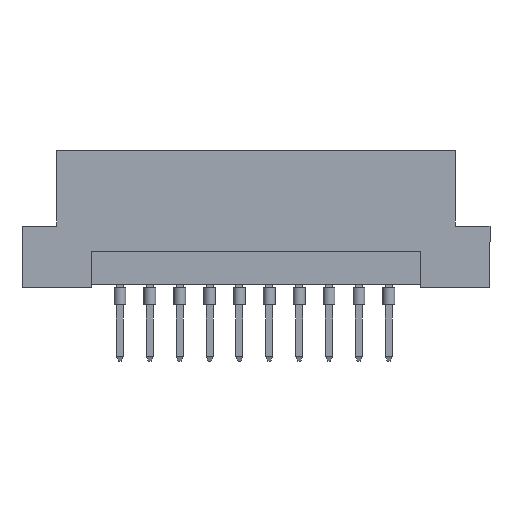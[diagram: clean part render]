
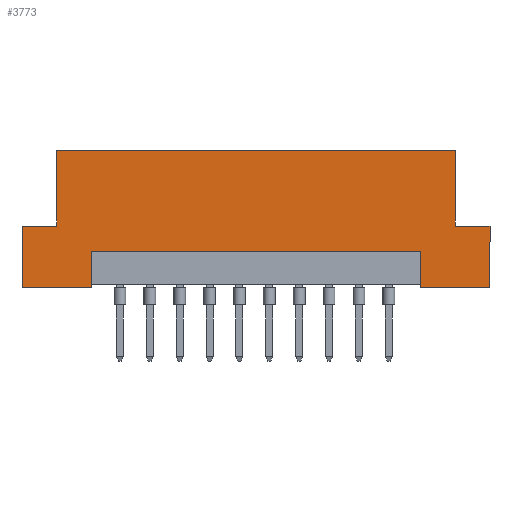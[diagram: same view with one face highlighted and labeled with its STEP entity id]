
A CAD part, front view. The second image highlights one B-rep face of the part: STEP entity #3773.
In plain terms, the highlighted planar face has unit normal (0, -1, 0).
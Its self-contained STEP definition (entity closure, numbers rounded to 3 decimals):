
#22 = VECTOR ( 'NONE', #2826, 1000. ) ;
#54 = LINE ( 'NONE', #463, #5178 ) ;
#62 = DIRECTION ( 'NONE',  ( 1., 0., 0. ) ) ;
#83 = ORIENTED_EDGE ( 'NONE', *, *, #1133, .F. ) ;
#179 = EDGE_CURVE ( 'NONE', #1130, #1898, #4204, .T. ) ;
#191 = ORIENTED_EDGE ( 'NONE', *, *, #2195, .T. ) ;
#226 = DIRECTION ( 'NONE',  ( 0., 0., 1. ) ) ;
#286 = CARTESIAN_POINT ( 'NONE',  ( 16.94, -4.3, 5.2 ) ) ;
#406 = VERTEX_POINT ( 'NONE', #3830 ) ;
#463 = CARTESIAN_POINT ( 'NONE',  ( 19.9, -4.3, 11.6 ) ) ;
#523 = EDGE_CURVE ( 'NONE', #3081, #2697, #657, .T. ) ;
#524 = DIRECTION ( 'NONE',  ( 1., 0., 0. ) ) ;
#594 = DIRECTION ( 'NONE',  ( 0., 0., -1. ) ) ;
#620 = ORIENTED_EDGE ( 'NONE', *, *, #4673, .F. ) ;
#657 = LINE ( 'NONE', #4878, #22 ) ;
#660 = CARTESIAN_POINT ( 'NONE',  ( 19.9, -4.3, 5.2 ) ) ;
#670 = DIRECTION ( 'NONE',  ( 0., 0., -1. ) ) ;
#687 = CARTESIAN_POINT ( 'NONE',  ( 14., -4.3, 3. ) ) ;
#706 = CARTESIAN_POINT ( 'NONE',  ( -14., -4.3, 3. ) ) ;
#811 = CARTESIAN_POINT ( 'NONE',  ( -19.9, -4.3, 11.6 ) ) ;
#885 = VECTOR ( 'NONE', #62, 1000. ) ;
#915 = CARTESIAN_POINT ( 'NONE',  ( -19.9, -4.3, 5.2 ) ) ;
#1026 = ORIENTED_EDGE ( 'NONE', *, *, #4464, .F. ) ;
#1111 = VECTOR ( 'NONE', #5130, 1000. ) ;
#1130 = VERTEX_POINT ( 'NONE', #2294 ) ;
#1133 = EDGE_CURVE ( 'NONE', #4198, #1898, #3945, .T. ) ;
#1314 = ORIENTED_EDGE ( 'NONE', *, *, #4512, .T. ) ;
#1452 = CARTESIAN_POINT ( 'NONE',  ( -14., -4.3, 3. ) ) ;
#1474 = CARTESIAN_POINT ( 'NONE',  ( -14., -4.3, 0.2 ) ) ;
#1511 = EDGE_LOOP ( 'NONE', ( #2979, #620, #3837, #4017, #2595, #1314, #2656, #1026, #4530, #191, #2821, #83 ) ) ;
#1546 = VECTOR ( 'NONE', #2391, 1000. ) ;
#1682 = LINE ( 'NONE', #4716, #4160 ) ;
#1689 = VERTEX_POINT ( 'NONE', #286 ) ;
#1718 = DIRECTION ( 'NONE',  ( 1., 0., 0. ) ) ;
#1791 = CARTESIAN_POINT ( 'NONE',  ( -14., -4.3, 0. ) ) ;
#1898 = VERTEX_POINT ( 'NONE', #1791 ) ;
#1913 = VECTOR ( 'NONE', #2459, 1000. ) ;
#1931 = EDGE_CURVE ( 'NONE', #1689, #4643, #1682, .T. ) ;
#2195 = EDGE_CURVE ( 'NONE', #5096, #1130, #4946, .T. ) ;
#2254 = DIRECTION ( 'NONE',  ( 1., 0., 0. ) ) ;
#2269 = LINE ( 'NONE', #4709, #4513 ) ;
#2283 = PLANE ( 'NONE',  #5342 ) ;
#2294 = CARTESIAN_POINT ( 'NONE',  ( -19.9, -4.3, 0. ) ) ;
#2307 = VECTOR ( 'NONE', #1718, 1000. ) ;
#2391 = DIRECTION ( 'NONE',  ( 0., 0., 1. ) ) ;
#2453 = EDGE_CURVE ( 'NONE', #4643, #2697, #2269, .T. ) ;
#2459 = DIRECTION ( 'NONE',  ( 0., 0., -1. ) ) ;
#2559 = CARTESIAN_POINT ( 'NONE',  ( -19.9, -4.3, 5.2 ) ) ;
#2595 = ORIENTED_EDGE ( 'NONE', *, *, #1931, .F. ) ;
#2656 = ORIENTED_EDGE ( 'NONE', *, *, #4054, .F. ) ;
#2697 = VERTEX_POINT ( 'NONE', #3244 ) ;
#2724 = EDGE_CURVE ( 'NONE', #5096, #3654, #3754, .T. ) ;
#2821 = ORIENTED_EDGE ( 'NONE', *, *, #179, .T. ) ;
#2826 = DIRECTION ( 'NONE',  ( 1., 0., 0. ) ) ;
#2829 = CARTESIAN_POINT ( 'NONE',  ( 16.94, -4.3, 11.6 ) ) ;
#2979 = ORIENTED_EDGE ( 'NONE', *, *, #3908, .T. ) ;
#3027 = CARTESIAN_POINT ( 'NONE',  ( 16.94, -4.3, 5.2 ) ) ;
#3081 = VERTEX_POINT ( 'NONE', #4157 ) ;
#3154 = DIRECTION ( 'NONE',  ( 0., 1., 0. ) ) ;
#3167 = DIRECTION ( 'NONE',  ( 1., 0., 0. ) ) ;
#3244 = CARTESIAN_POINT ( 'NONE',  ( 19.9, -4.3, 0. ) ) ;
#3277 = VECTOR ( 'NONE', #3167, 1000. ) ;
#3519 = LINE ( 'NONE', #1452, #3277 ) ;
#3533 = CARTESIAN_POINT ( 'NONE',  ( 19.9, -4.3, 11.6 ) ) ;
#3535 = LINE ( 'NONE', #3027, #1111 ) ;
#3654 = VERTEX_POINT ( 'NONE', #4823 ) ;
#3710 = VERTEX_POINT ( 'NONE', #687 ) ;
#3754 = LINE ( 'NONE', #2559, #2307 ) ;
#3773 = ADVANCED_FACE ( 'NONE', ( #4337 ), #2283, .F. ) ;
#3830 = CARTESIAN_POINT ( 'NONE',  ( -16.94, -4.3, 11.6 ) ) ;
#3834 = LINE ( 'NONE', #4646, #5097 ) ;
#3837 = ORIENTED_EDGE ( 'NONE', *, *, #523, .T. ) ;
#3908 = EDGE_CURVE ( 'NONE', #4198, #3710, #3519, .T. ) ;
#3945 = LINE ( 'NONE', #1474, #4516 ) ;
#4017 = ORIENTED_EDGE ( 'NONE', *, *, #2453, .F. ) ;
#4054 = EDGE_CURVE ( 'NONE', #406, #4619, #54, .T. ) ;
#4157 = CARTESIAN_POINT ( 'NONE',  ( 14., -4.3, 0. ) ) ;
#4160 = VECTOR ( 'NONE', #2254, 1000. ) ;
#4198 = VERTEX_POINT ( 'NONE', #706 ) ;
#4204 = LINE ( 'NONE', #5340, #885 ) ;
#4337 = FACE_OUTER_BOUND ( 'NONE', #1511, .T. ) ;
#4464 = EDGE_CURVE ( 'NONE', #3654, #406, #3834, .T. ) ;
#4512 = EDGE_CURVE ( 'NONE', #1689, #4619, #3535, .T. ) ;
#4513 = VECTOR ( 'NONE', #594, 1000. ) ;
#4516 = VECTOR ( 'NONE', #670, 1000. ) ;
#4530 = ORIENTED_EDGE ( 'NONE', *, *, #2724, .F. ) ;
#4619 = VERTEX_POINT ( 'NONE', #2829 ) ;
#4643 = VERTEX_POINT ( 'NONE', #660 ) ;
#4646 = CARTESIAN_POINT ( 'NONE',  ( -16.94, -4.3, 5.2 ) ) ;
#4673 = EDGE_CURVE ( 'NONE', #3081, #3710, #5232, .T. ) ;
#4709 = CARTESIAN_POINT ( 'NONE',  ( 19.9, -4.3, 11.6 ) ) ;
#4716 = CARTESIAN_POINT ( 'NONE',  ( 19.9, -4.3, 5.2 ) ) ;
#4823 = CARTESIAN_POINT ( 'NONE',  ( -16.94, -4.3, 5.2 ) ) ;
#4827 = CARTESIAN_POINT ( 'NONE',  ( 14., -4.3, 0.2 ) ) ;
#4878 = CARTESIAN_POINT ( 'NONE',  ( 19.9, -4.3, 0. ) ) ;
#4946 = LINE ( 'NONE', #811, #1913 ) ;
#5096 = VERTEX_POINT ( 'NONE', #915 ) ;
#5097 = VECTOR ( 'NONE', #226, 1000. ) ;
#5130 = DIRECTION ( 'NONE',  ( 0., 0., 1. ) ) ;
#5177 = DIRECTION ( 'NONE',  ( -1., 0., 0. ) ) ;
#5178 = VECTOR ( 'NONE', #524, 1000. ) ;
#5232 = LINE ( 'NONE', #4827, #1546 ) ;
#5340 = CARTESIAN_POINT ( 'NONE',  ( 19.9, -4.3, 0. ) ) ;
#5342 = AXIS2_PLACEMENT_3D ( 'NONE', #3533, #3154, #5177 ) ;
